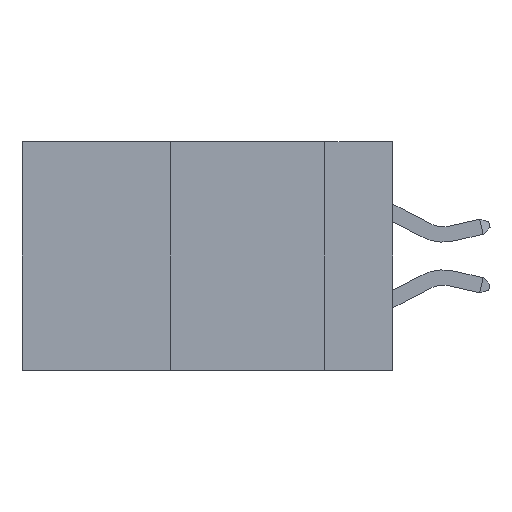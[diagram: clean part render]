
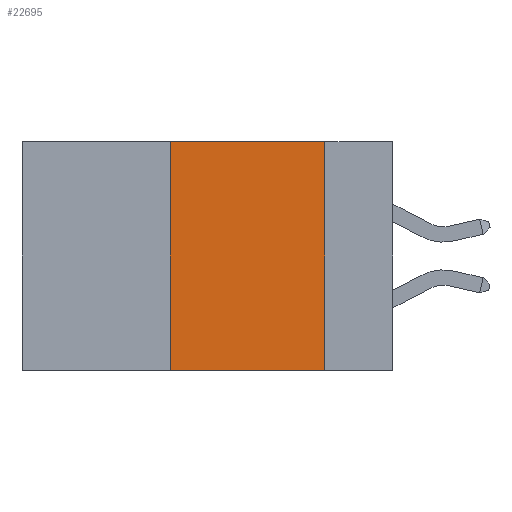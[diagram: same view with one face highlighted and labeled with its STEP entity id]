
A CAD part, left-side view. The second image highlights one B-rep face of the part: STEP entity #22695.
In plain terms, the highlighted planar face has unit normal (-1, 0, 0).
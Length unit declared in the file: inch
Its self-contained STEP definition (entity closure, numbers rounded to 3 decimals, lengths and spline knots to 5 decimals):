
#240 = EDGE_CURVE ( 'NONE', #21097, #34017, #13599, .T. ) ;
#1618 = FACE_OUTER_BOUND ( 'NONE', #3910, .T. ) ;
#2255 = ORIENTED_EDGE ( 'NONE', *, *, #240, .F. ) ;
#3141 = PLANE ( 'NONE',  #24800 ) ;
#3572 = CARTESIAN_POINT ( 'NONE',  ( 0., 0.6, -0.37 ) ) ;
#3910 = EDGE_LOOP ( 'NONE', ( #18512, #2255, #20970, #31768 ) ) ;
#6238 = DIRECTION ( 'NONE',  ( 1., 0., 0. ) ) ;
#7220 = DIRECTION ( 'NONE',  ( 0., 0., 1. ) ) ;
#9199 = EDGE_CURVE ( 'NONE', #34017, #31754, #21418, .T. ) ;
#12636 = VECTOR ( 'NONE', #31318, 39.37008 ) ;
#13320 = VECTOR ( 'NONE', #13703, 39.37008 ) ;
#13599 = LINE ( 'NONE', #36527, #12636 ) ;
#13703 = DIRECTION ( 'NONE',  ( 0., 0., -1. ) ) ;
#15137 = VECTOR ( 'NONE', #7220, 39.37008 ) ;
#15226 = CARTESIAN_POINT ( 'NONE',  ( 0., 0.11, 0. ) ) ;
#16273 = VERTEX_POINT ( 'NONE', #27905 ) ;
#16480 = CARTESIAN_POINT ( 'NONE',  ( 0., 0.36, 0. ) ) ;
#18512 = ORIENTED_EDGE ( 'NONE', *, *, #9199, .F. ) ;
#19383 = CARTESIAN_POINT ( 'NONE',  ( 0., 0.36, 0. ) ) ;
#20970 = ORIENTED_EDGE ( 'NONE', *, *, #39472, .F. ) ;
#21097 = VERTEX_POINT ( 'NONE', #16480 ) ;
#21418 = LINE ( 'NONE', #35114, #13320 ) ;
#21896 = DIRECTION ( 'NONE',  ( 0., -1., 0. ) ) ;
#22247 = EDGE_CURVE ( 'NONE', #16273, #31754, #35739, .T. ) ;
#22288 = LINE ( 'NONE', #19383, #15137 ) ;
#22450 = CARTESIAN_POINT ( 'NONE',  ( 0., 0.11, -0.37 ) ) ;
#22695 = ADVANCED_FACE ( 'NONE', ( #1618 ), #3141, .F. ) ;
#24800 = AXIS2_PLACEMENT_3D ( 'NONE', #36776, #6238, #27669 ) ;
#27669 = DIRECTION ( 'NONE',  ( 0., 0., -1. ) ) ;
#27905 = CARTESIAN_POINT ( 'NONE',  ( 0., 0.36, -0.37 ) ) ;
#28552 = VECTOR ( 'NONE', #21896, 39.37008 ) ;
#31318 = DIRECTION ( 'NONE',  ( 0., -1., 0. ) ) ;
#31754 = VERTEX_POINT ( 'NONE', #22450 ) ;
#31768 = ORIENTED_EDGE ( 'NONE', *, *, #22247, .T. ) ;
#34017 = VERTEX_POINT ( 'NONE', #15226 ) ;
#35114 = CARTESIAN_POINT ( 'NONE',  ( 0., 0.11, 0. ) ) ;
#35739 = LINE ( 'NONE', #3572, #28552 ) ;
#36527 = CARTESIAN_POINT ( 'NONE',  ( 0., 0.6, 0. ) ) ;
#36776 = CARTESIAN_POINT ( 'NONE',  ( 0., 0.6, 0. ) ) ;
#39472 = EDGE_CURVE ( 'NONE', #16273, #21097, #22288, .T. ) ;
